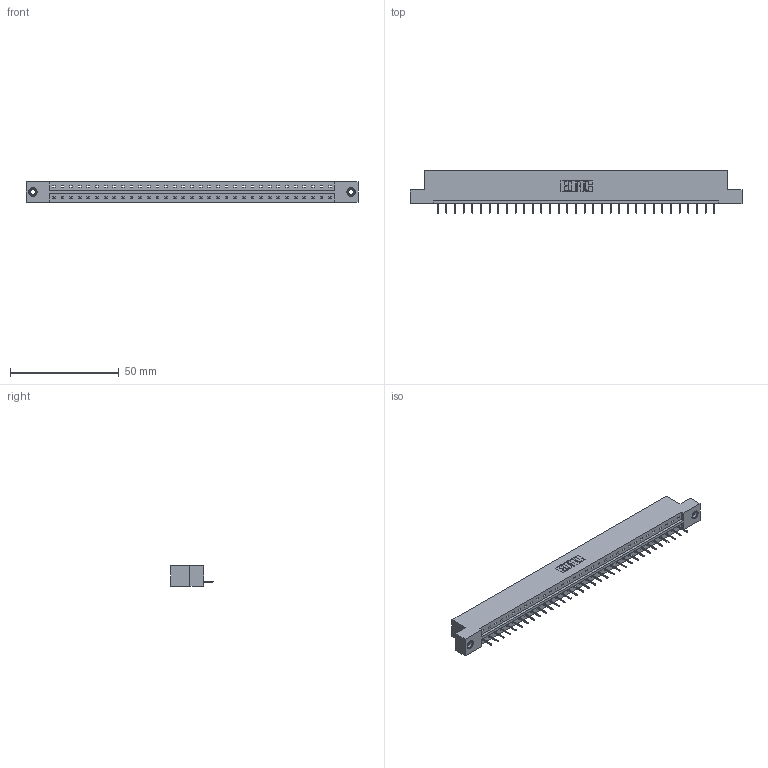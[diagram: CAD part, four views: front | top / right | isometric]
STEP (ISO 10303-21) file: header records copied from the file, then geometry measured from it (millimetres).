
FILE_DESCRIPTION (( 'STEP AP203' ), '1' );
FILE_NAME ('333-033-524-108.STEP', '2018-08-02T21:10:30', ( '' ), ( '' ), 'SwSTEP 2.0', 'SolidWorks 2016', '' );
FILE_SCHEMA (( 'CONFIG_CONTROL_DESIGN' ));
Length unit declared in the file: inch
Products named in the file (4): 333 Part_Flush - .156 Dia - TI; 345-292-001_345-293-124; 345-250-001_345-250-003-102; 333-033-524-108
Assembly tree (36 placements, depth 2):
  333-033-524-108
    333 Part_Flush - .156 Dia - TI
    345-292-001_345-293-124  x33
    345-250-001_345-250-003-102  x2
Bounding box: 152.3 x 19.69 x 9.4 mm (x, y, z)
Volume: 15111.2 mm3; surface area: 15869.1 mm2
Topology: 36 solids, 36 shells, 2220 faces, 6387 edges, 4118 vertices
Faces by surface type: plane 1686, cylinder 518, cone 12, torus 4
Entity records: 22598 total; most frequent: CARTESIAN_POINT 3880, ORIENTED_EDGE 3842, DIRECTION 3325, EDGE_CURVE 1921, VECTOR 1777, LINE 1777, VERTEX_POINT 1272, AXIS2_PLACEMENT_3D 774
